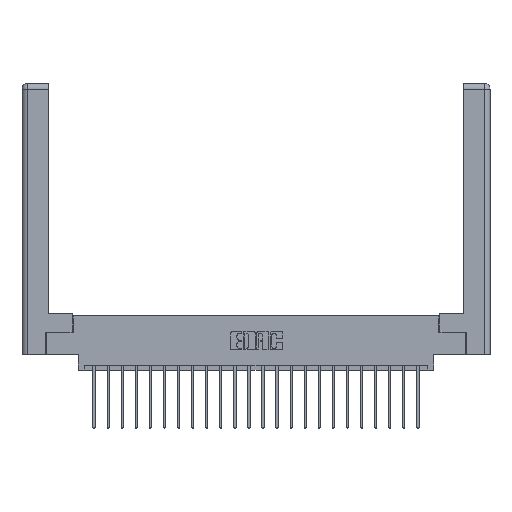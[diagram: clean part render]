
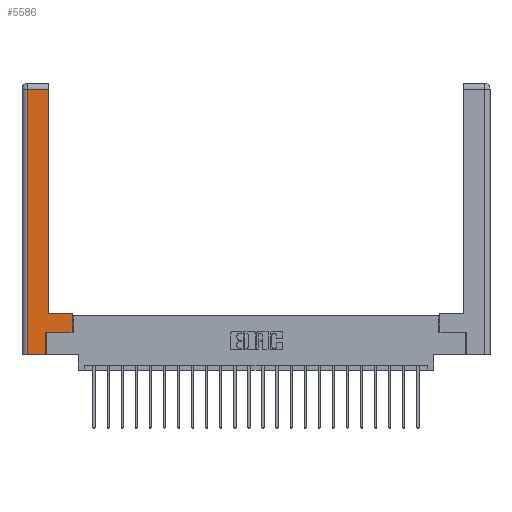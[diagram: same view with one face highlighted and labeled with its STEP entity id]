
A CAD part, top view. The second image highlights one B-rep face of the part: STEP entity #5586.
In plain terms, the highlighted planar face has unit normal (0, 0, 1).
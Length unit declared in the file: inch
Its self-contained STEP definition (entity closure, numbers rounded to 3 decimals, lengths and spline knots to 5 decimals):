
#115 = VERTEX_POINT ( 'NONE', #13452 ) ;
#491 = ORIENTED_EDGE ( 'NONE', *, *, #20575, .T. ) ;
#732 = ORIENTED_EDGE ( 'NONE', *, *, #6235, .T. ) ;
#986 = FACE_OUTER_BOUND ( 'NONE', #21249, .T. ) ;
#1342 = CARTESIAN_POINT ( 'NONE',  ( 0.0615, 2.94, 0. ) ) ;
#1427 = VECTOR ( 'NONE', #23360, 39.37008 ) ;
#1707 = LINE ( 'NONE', #15928, #1427 ) ;
#2450 = EDGE_CURVE ( 'NONE', #12902, #115, #8414, .T. ) ;
#2959 = LINE ( 'NONE', #16960, #22734 ) ;
#3421 = ORIENTED_EDGE ( 'NONE', *, *, #6311, .T. ) ;
#3979 = EDGE_CURVE ( 'NONE', #6543, #14362, #4926, .T. ) ;
#4926 = LINE ( 'NONE', #7704, #8076 ) ;
#5277 = LINE ( 'NONE', #1342, #8701 ) ;
#5586 = ADVANCED_FACE ( 'NONE', ( #986 ), #21162, .F. ) ;
#5606 = VERTEX_POINT ( 'NONE', #8030 ) ;
#5759 = ORIENTED_EDGE ( 'NONE', *, *, #3979, .T. ) ;
#6107 = VECTOR ( 'NONE', #11165, 39.37008 ) ;
#6235 = EDGE_CURVE ( 'NONE', #5606, #12513, #10990, .T. ) ;
#6311 = EDGE_CURVE ( 'NONE', #21597, #12902, #2959, .T. ) ;
#6543 = VERTEX_POINT ( 'NONE', #13864 ) ;
#6682 = VECTOR ( 'NONE', #17282, 39.37008 ) ;
#6750 = ORIENTED_EDGE ( 'NONE', *, *, #9083, .T. ) ;
#7562 = AXIS2_PLACEMENT_3D ( 'NONE', #13953, #23300, #13874 ) ;
#7704 = CARTESIAN_POINT ( 'NONE',  ( 0.295, 0.45, 0. ) ) ;
#8030 = CARTESIAN_POINT ( 'NONE',  ( 0.265, 0.245, 0. ) ) ;
#8076 = VECTOR ( 'NONE', #11265, 39.37008 ) ;
#8414 = LINE ( 'NONE', #10123, #6682 ) ;
#8551 = VECTOR ( 'NONE', #23003, 39.37008 ) ;
#8701 = VECTOR ( 'NONE', #12357, 39.37008 ) ;
#9083 = EDGE_CURVE ( 'NONE', #14362, #10542, #10288, .T. ) ;
#10123 = CARTESIAN_POINT ( 'NONE',  ( 0.265, 0., 0. ) ) ;
#10288 = LINE ( 'NONE', #19310, #8551 ) ;
#10542 = VERTEX_POINT ( 'NONE', #18339 ) ;
#10990 = LINE ( 'NONE', #20253, #6107 ) ;
#11165 = DIRECTION ( 'NONE',  ( 1., 0., 0. ) ) ;
#11265 = DIRECTION ( 'NONE',  ( -1., 0., 0. ) ) ;
#12101 = CARTESIAN_POINT ( 'NONE',  ( 0.0615, 0., 0. ) ) ;
#12357 = DIRECTION ( 'NONE',  ( -1., 0., 0. ) ) ;
#12513 = VERTEX_POINT ( 'NONE', #13925 ) ;
#12546 = VECTOR ( 'NONE', #20778, 39.37008 ) ;
#12902 = VERTEX_POINT ( 'NONE', #12101 ) ;
#13452 = CARTESIAN_POINT ( 'NONE',  ( 0.265, 0., 0. ) ) ;
#13864 = CARTESIAN_POINT ( 'NONE',  ( 0.565, 0.45, 0. ) ) ;
#13874 = DIRECTION ( 'NONE',  ( -1., 0., 0. ) ) ;
#13925 = CARTESIAN_POINT ( 'NONE',  ( 0.565, 0.245, 0. ) ) ;
#13953 = CARTESIAN_POINT ( 'NONE',  ( 0., 0., 0. ) ) ;
#14362 = VERTEX_POINT ( 'NONE', #19270 ) ;
#14612 = ORIENTED_EDGE ( 'NONE', *, *, #18304, .T. ) ;
#15158 = CARTESIAN_POINT ( 'NONE',  ( 0.0615, 2.94, 0. ) ) ;
#15294 = DIRECTION ( 'NONE',  ( 0., -1., 0. ) ) ;
#15928 = CARTESIAN_POINT ( 'NONE',  ( 0.265, 0.245, 0. ) ) ;
#16341 = EDGE_CURVE ( 'NONE', #12513, #6543, #17356, .T. ) ;
#16960 = CARTESIAN_POINT ( 'NONE',  ( 0.0615, 0., 0. ) ) ;
#17282 = DIRECTION ( 'NONE',  ( 1., 0., 0. ) ) ;
#17356 = LINE ( 'NONE', #18758, #12546 ) ;
#18304 = EDGE_CURVE ( 'NONE', #10542, #21597, #5277, .T. ) ;
#18339 = CARTESIAN_POINT ( 'NONE',  ( 0.295, 2.94, 0. ) ) ;
#18758 = CARTESIAN_POINT ( 'NONE',  ( 0.565, 0.45, 0. ) ) ;
#18767 = ORIENTED_EDGE ( 'NONE', *, *, #2450, .T. ) ;
#19270 = CARTESIAN_POINT ( 'NONE',  ( 0.295, 0.45, 0. ) ) ;
#19310 = CARTESIAN_POINT ( 'NONE',  ( 0.295, 3., 0. ) ) ;
#20253 = CARTESIAN_POINT ( 'NONE',  ( 0.565, 0.245, 0. ) ) ;
#20575 = EDGE_CURVE ( 'NONE', #115, #5606, #1707, .T. ) ;
#20778 = DIRECTION ( 'NONE',  ( 0., 1., 0. ) ) ;
#21162 = PLANE ( 'NONE',  #7562 ) ;
#21249 = EDGE_LOOP ( 'NONE', ( #6750, #14612, #3421, #18767, #491, #732, #22344, #5759 ) ) ;
#21597 = VERTEX_POINT ( 'NONE', #15158 ) ;
#22344 = ORIENTED_EDGE ( 'NONE', *, *, #16341, .T. ) ;
#22734 = VECTOR ( 'NONE', #15294, 39.37008 ) ;
#23003 = DIRECTION ( 'NONE',  ( 0., 1., 0. ) ) ;
#23300 = DIRECTION ( 'NONE',  ( 0., 0., -1. ) ) ;
#23360 = DIRECTION ( 'NONE',  ( 0., 1., 0. ) ) ;
